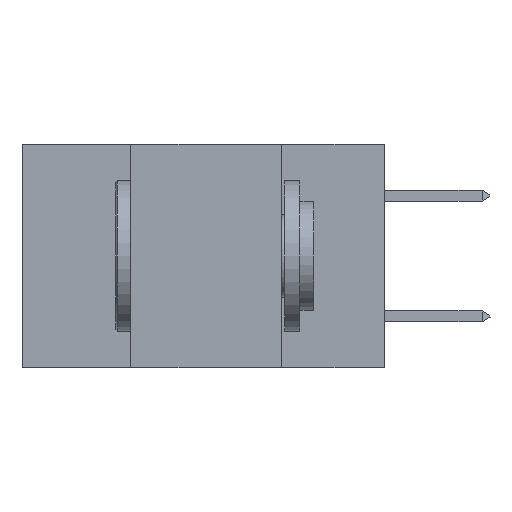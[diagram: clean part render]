
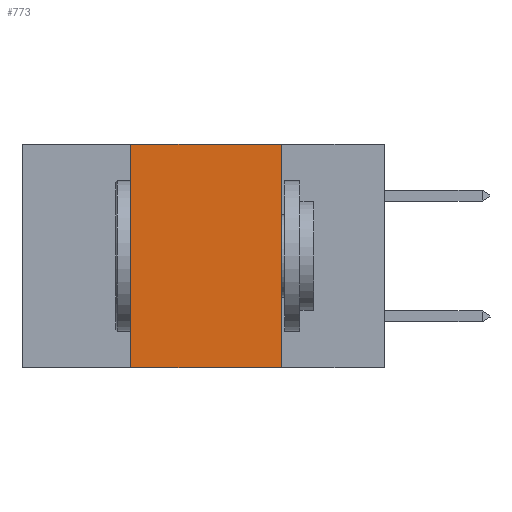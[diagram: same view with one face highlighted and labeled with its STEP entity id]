
A CAD part, left-side view. The second image highlights one B-rep face of the part: STEP entity #773.
In plain terms, the highlighted planar face has unit normal (-1, 0, 0).
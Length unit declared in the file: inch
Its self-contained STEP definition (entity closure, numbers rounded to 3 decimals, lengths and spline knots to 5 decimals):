
#201 = LINE ( 'NONE', #16393, #9061 ) ;
#773 = ADVANCED_FACE ( 'NONE', ( #13865 ), #11229, .F. ) ;
#850 = EDGE_CURVE ( 'NONE', #14947, #7783, #22017, .T. ) ;
#1055 = DIRECTION ( 'NONE',  ( 0., 0., -1. ) ) ;
#3798 = DIRECTION ( 'NONE',  ( 0., 0., -1. ) ) ;
#3966 = VERTEX_POINT ( 'NONE', #21829 ) ;
#4024 = LINE ( 'NONE', #14347, #4595 ) ;
#4595 = VECTOR ( 'NONE', #1055, 39.37008 ) ;
#4852 = CARTESIAN_POINT ( 'NONE',  ( 0., 0.6, 0. ) ) ;
#4899 = CARTESIAN_POINT ( 'NONE',  ( 0., 0.17, 0. ) ) ;
#5174 = CARTESIAN_POINT ( 'NONE',  ( 0., 0.42, 0. ) ) ;
#6525 = ORIENTED_EDGE ( 'NONE', *, *, #850, .F. ) ;
#6571 = CARTESIAN_POINT ( 'NONE',  ( 0., 0.42, -0.37 ) ) ;
#7783 = VERTEX_POINT ( 'NONE', #4899 ) ;
#8095 = ORIENTED_EDGE ( 'NONE', *, *, #13448, .F. ) ;
#9061 = VECTOR ( 'NONE', #23592, 39.37008 ) ;
#9456 = ORIENTED_EDGE ( 'NONE', *, *, #23175, .T. ) ;
#9475 = CARTESIAN_POINT ( 'NONE',  ( 0., 0.42, 0. ) ) ;
#9972 = LINE ( 'NONE', #5174, #10282 ) ;
#9986 = ORIENTED_EDGE ( 'NONE', *, *, #21924, .F. ) ;
#10282 = VECTOR ( 'NONE', #12568, 39.37008 ) ;
#11229 = PLANE ( 'NONE',  #12494 ) ;
#12494 = AXIS2_PLACEMENT_3D ( 'NONE', #20446, #22414, #3798 ) ;
#12568 = DIRECTION ( 'NONE',  ( 0., 0., 1. ) ) ;
#13448 = EDGE_CURVE ( 'NONE', #7783, #3966, #4024, .T. ) ;
#13865 = FACE_OUTER_BOUND ( 'NONE', #21577, .T. ) ;
#14347 = CARTESIAN_POINT ( 'NONE',  ( 0., 0.17, 0. ) ) ;
#14947 = VERTEX_POINT ( 'NONE', #9475 ) ;
#15110 = DIRECTION ( 'NONE',  ( 0., -1., 0. ) ) ;
#16393 = CARTESIAN_POINT ( 'NONE',  ( 0., 0.6, -0.37 ) ) ;
#17051 = VERTEX_POINT ( 'NONE', #6571 ) ;
#20446 = CARTESIAN_POINT ( 'NONE',  ( 0., 0.6, 0. ) ) ;
#21140 = VECTOR ( 'NONE', #15110, 39.37008 ) ;
#21577 = EDGE_LOOP ( 'NONE', ( #8095, #6525, #9986, #9456 ) ) ;
#21829 = CARTESIAN_POINT ( 'NONE',  ( 0., 0.17, -0.37 ) ) ;
#21924 = EDGE_CURVE ( 'NONE', #17051, #14947, #9972, .T. ) ;
#22017 = LINE ( 'NONE', #4852, #21140 ) ;
#22414 = DIRECTION ( 'NONE',  ( 1., 0., 0. ) ) ;
#23175 = EDGE_CURVE ( 'NONE', #17051, #3966, #201, .T. ) ;
#23592 = DIRECTION ( 'NONE',  ( 0., -1., 0. ) ) ;
